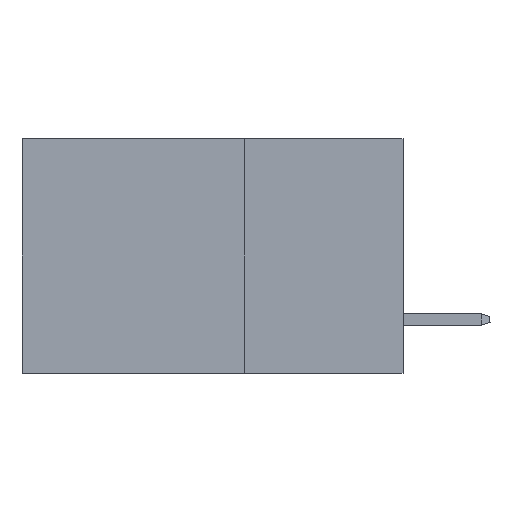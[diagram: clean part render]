
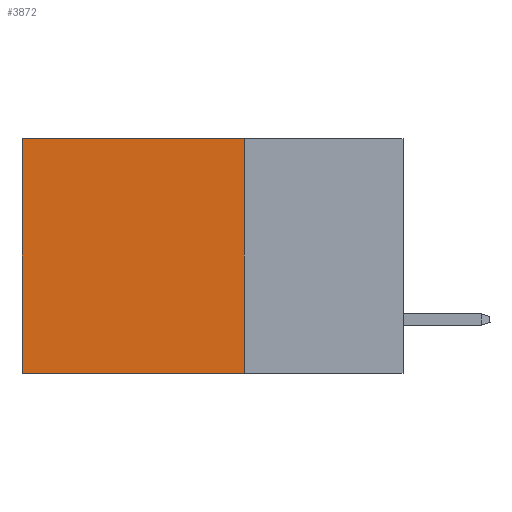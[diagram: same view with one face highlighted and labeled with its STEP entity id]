
A CAD part, left-side view. The second image highlights one B-rep face of the part: STEP entity #3872.
In plain terms, the highlighted planar face has unit normal (-1, 0, 0).
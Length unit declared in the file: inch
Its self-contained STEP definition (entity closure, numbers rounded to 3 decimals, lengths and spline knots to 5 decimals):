
#359 = VECTOR ( 'NONE', #27145, 39.37008 ) ;
#645 = CARTESIAN_POINT ( 'NONE',  ( 0.2875, 0.6, -0.37 ) ) ;
#1189 = ORIENTED_EDGE ( 'NONE', *, *, #21725, .F. ) ;
#3205 = CARTESIAN_POINT ( 'NONE',  ( 0.2875, 0.25, 0. ) ) ;
#3521 = DIRECTION ( 'NONE',  ( 0., 0., -1. ) ) ;
#3872 = ADVANCED_FACE ( 'NONE', ( #9417 ), #13838, .F. ) ;
#4705 = VECTOR ( 'NONE', #24424, 39.37008 ) ;
#5558 = CARTESIAN_POINT ( 'NONE',  ( 0.2875, 0.25, -0.37 ) ) ;
#7325 = EDGE_CURVE ( 'NONE', #20222, #8960, #9438, .T. ) ;
#7643 = CARTESIAN_POINT ( 'NONE',  ( 0.2875, 0.25, 0. ) ) ;
#7983 = ORIENTED_EDGE ( 'NONE', *, *, #22564, .T. ) ;
#8960 = VERTEX_POINT ( 'NONE', #645 ) ;
#9417 = FACE_OUTER_BOUND ( 'NONE', #9880, .T. ) ;
#9438 = LINE ( 'NONE', #5558, #20028 ) ;
#9880 = EDGE_LOOP ( 'NONE', ( #7983, #16611, #1189, #14847 ) ) ;
#11628 = DIRECTION ( 'NONE',  ( 1., 0., 0. ) ) ;
#11646 = DIRECTION ( 'NONE',  ( 0., 1., 0. ) ) ;
#11855 = LINE ( 'NONE', #16137, #4705 ) ;
#11964 = LINE ( 'NONE', #20271, #359 ) ;
#12998 = VERTEX_POINT ( 'NONE', #25358 ) ;
#13498 = VECTOR ( 'NONE', #3521, 39.37008 ) ;
#13838 = PLANE ( 'NONE',  #24789 ) ;
#14021 = LINE ( 'NONE', #20250, #13498 ) ;
#14847 = ORIENTED_EDGE ( 'NONE', *, *, #26495, .T. ) ;
#16137 = CARTESIAN_POINT ( 'NONE',  ( 0.2875, 0.6, 0. ) ) ;
#16611 = ORIENTED_EDGE ( 'NONE', *, *, #7325, .F. ) ;
#20028 = VECTOR ( 'NONE', #11646, 39.37008 ) ;
#20222 = VERTEX_POINT ( 'NONE', #25607 ) ;
#20250 = CARTESIAN_POINT ( 'NONE',  ( 0.2875, 0.25, 0. ) ) ;
#20271 = CARTESIAN_POINT ( 'NONE',  ( 0.2875, 0.25, 0. ) ) ;
#21725 = EDGE_CURVE ( 'NONE', #23459, #20222, #14021, .T. ) ;
#22265 = DIRECTION ( 'NONE',  ( 0., 0., -1. ) ) ;
#22564 = EDGE_CURVE ( 'NONE', #12998, #8960, #11855, .T. ) ;
#23459 = VERTEX_POINT ( 'NONE', #7643 ) ;
#24424 = DIRECTION ( 'NONE',  ( 0., 0., -1. ) ) ;
#24789 = AXIS2_PLACEMENT_3D ( 'NONE', #3205, #11628, #22265 ) ;
#25358 = CARTESIAN_POINT ( 'NONE',  ( 0.2875, 0.6, 0. ) ) ;
#25607 = CARTESIAN_POINT ( 'NONE',  ( 0.2875, 0.25, -0.37 ) ) ;
#26495 = EDGE_CURVE ( 'NONE', #23459, #12998, #11964, .T. ) ;
#27145 = DIRECTION ( 'NONE',  ( 0., 1., 0. ) ) ;
